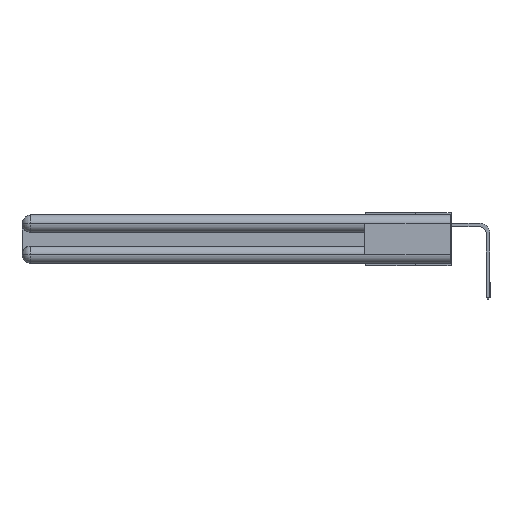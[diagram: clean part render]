
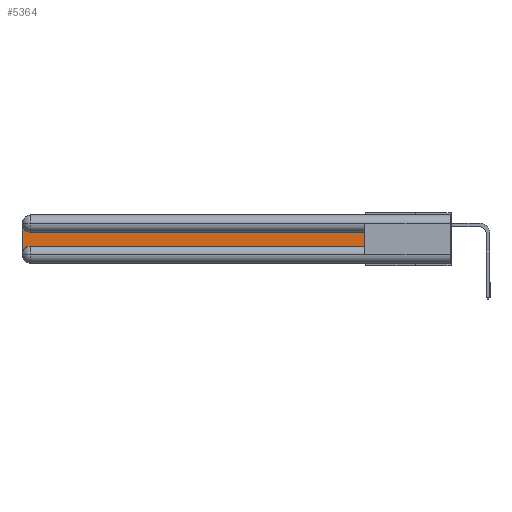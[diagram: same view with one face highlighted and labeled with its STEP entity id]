
A CAD part, left-side view. The second image highlights one B-rep face of the part: STEP entity #5364.
In plain terms, the highlighted planar face has unit normal (-1, 0, 0).
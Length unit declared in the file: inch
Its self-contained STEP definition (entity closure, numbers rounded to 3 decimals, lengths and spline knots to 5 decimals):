
#2009 = VECTOR ( 'NONE', #14086, 39.37008 ) ;
#2127 = DIRECTION ( 'NONE',  ( 1., 0., 0. ) ) ;
#2389 = CARTESIAN_POINT ( 'NONE',  ( 0.075, 3., -0.2175 ) ) ;
#2467 = VECTOR ( 'NONE', #20145, 39.37008 ) ;
#2607 = CARTESIAN_POINT ( 'NONE',  ( 0.075, 3., -0.0625 ) ) ;
#2937 = DIRECTION ( 'NONE',  ( 1., 0., 0. ) ) ;
#3623 = LINE ( 'NONE', #29391, #2009 ) ;
#4266 = ORIENTED_EDGE ( 'NONE', *, *, #9039, .T. ) ;
#4703 = ORIENTED_EDGE ( 'NONE', *, *, #11750, .T. ) ;
#4772 = EDGE_LOOP ( 'NONE', ( #26800, #32721, #26859, #17280, #4703, #4266 ) ) ;
#4958 = DIRECTION ( 'NONE',  ( 0., 0., -1. ) ) ;
#5364 = ADVANCED_FACE ( 'NONE', ( #28042 ), #13047, .F. ) ;
#7074 = AXIS2_PLACEMENT_3D ( 'NONE', #27931, #2127, #4958 ) ;
#7112 = VECTOR ( 'NONE', #29978, 39.37008 ) ;
#7213 = VERTEX_POINT ( 'NONE', #26860 ) ;
#8125 = AXIS2_PLACEMENT_3D ( 'NONE', #17264, #30308, #14703 ) ;
#8915 = CARTESIAN_POINT ( 'NONE',  ( 0.075, 2.94, -0.2175 ) ) ;
#9039 = EDGE_CURVE ( 'NONE', #7213, #25745, #3623, .T. ) ;
#9560 = VERTEX_POINT ( 'NONE', #20457 ) ;
#9670 = AXIS2_PLACEMENT_3D ( 'NONE', #18236, #2937, #10687 ) ;
#10122 = CARTESIAN_POINT ( 'NONE',  ( 0.075, 0.6, -0.2175 ) ) ;
#10687 = DIRECTION ( 'NONE',  ( 0., 0., -1. ) ) ;
#11120 = CARTESIAN_POINT ( 'NONE',  ( 0.075, 3., -0.2775 ) ) ;
#11750 = EDGE_CURVE ( 'NONE', #25683, #7213, #30211, .T. ) ;
#13047 = PLANE ( 'NONE',  #9670 ) ;
#14086 = DIRECTION ( 'NONE',  ( 0., 0., 1. ) ) ;
#14441 = LINE ( 'NONE', #2389, #31350 ) ;
#14703 = DIRECTION ( 'NONE',  ( 0., 0., -1. ) ) ;
#17264 = CARTESIAN_POINT ( 'NONE',  ( 0.075, 2.94, -0.0625 ) ) ;
#17280 = ORIENTED_EDGE ( 'NONE', *, *, #29668, .T. ) ;
#18236 = CARTESIAN_POINT ( 'NONE',  ( 0.075, 3., -0.1225 ) ) ;
#19822 = EDGE_CURVE ( 'NONE', #25745, #9560, #25596, .T. ) ;
#19880 = CARTESIAN_POINT ( 'NONE',  ( 0.075, 0.6, -0.1225 ) ) ;
#20145 = DIRECTION ( 'NONE',  ( 0., -1., 0. ) ) ;
#20457 = CARTESIAN_POINT ( 'NONE',  ( 0.075, 2.94, -0.1225 ) ) ;
#20509 = DIRECTION ( 'NONE',  ( 0., 0., -1. ) ) ;
#21770 = CIRCLE ( 'NONE', #8125, 0.06 ) ;
#22055 = CARTESIAN_POINT ( 'NONE',  ( 0.075, 0.6, -0.1225 ) ) ;
#22567 = EDGE_CURVE ( 'NONE', #9560, #26507, #21770, .T. ) ;
#23280 = EDGE_CURVE ( 'NONE', #26507, #25715, #14441, .T. ) ;
#25596 = LINE ( 'NONE', #19880, #7112 ) ;
#25683 = VERTEX_POINT ( 'NONE', #8915 ) ;
#25715 = VERTEX_POINT ( 'NONE', #11120 ) ;
#25745 = VERTEX_POINT ( 'NONE', #22055 ) ;
#26507 = VERTEX_POINT ( 'NONE', #2607 ) ;
#26800 = ORIENTED_EDGE ( 'NONE', *, *, #19822, .T. ) ;
#26859 = ORIENTED_EDGE ( 'NONE', *, *, #23280, .T. ) ;
#26860 = CARTESIAN_POINT ( 'NONE',  ( 0.075, 0.6, -0.2175 ) ) ;
#27931 = CARTESIAN_POINT ( 'NONE',  ( 0.075, 2.94, -0.2775 ) ) ;
#28042 = FACE_OUTER_BOUND ( 'NONE', #4772, .T. ) ;
#29391 = CARTESIAN_POINT ( 'NONE',  ( 0.075, 0.6, -0.2175 ) ) ;
#29668 = EDGE_CURVE ( 'NONE', #25715, #25683, #30739, .T. ) ;
#29978 = DIRECTION ( 'NONE',  ( 0., 1., 0. ) ) ;
#30211 = LINE ( 'NONE', #10122, #2467 ) ;
#30308 = DIRECTION ( 'NONE',  ( 1., 0., 0. ) ) ;
#30739 = CIRCLE ( 'NONE', #7074, 0.06 ) ;
#31350 = VECTOR ( 'NONE', #20509, 39.37008 ) ;
#32721 = ORIENTED_EDGE ( 'NONE', *, *, #22567, .T. ) ;
